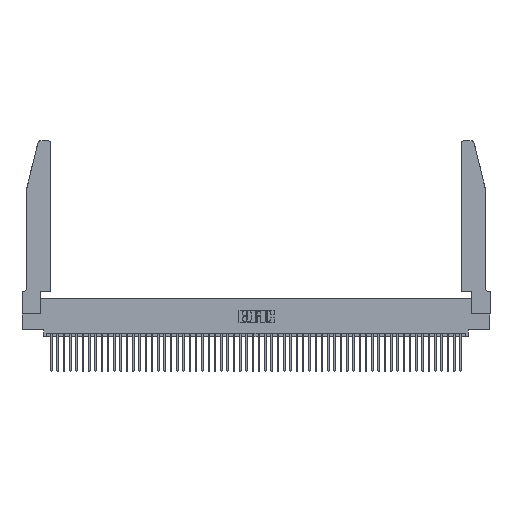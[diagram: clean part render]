
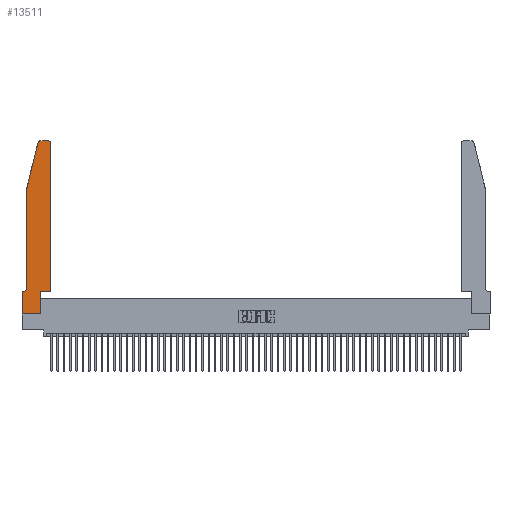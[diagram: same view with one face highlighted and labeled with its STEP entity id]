
A CAD part, top view. The second image highlights one B-rep face of the part: STEP entity #13511.
In plain terms, the highlighted planar face has unit normal (0, 0, 1).
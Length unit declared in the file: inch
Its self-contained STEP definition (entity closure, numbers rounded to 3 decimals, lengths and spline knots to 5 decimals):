
#61 = VECTOR ( 'NONE', #6870, 39.37008 ) ;
#768 = LINE ( 'NONE', #10422, #43506 ) ;
#879 = ORIENTED_EDGE ( 'NONE', *, *, #13769, .T. ) ;
#1245 = ORIENTED_EDGE ( 'NONE', *, *, #14559, .T. ) ;
#1617 = DIRECTION ( 'NONE',  ( 1., 0., 0. ) ) ;
#2369 = ORIENTED_EDGE ( 'NONE', *, *, #18976, .T. ) ;
#3714 = DIRECTION ( 'NONE',  ( 0., 0., 1. ) ) ;
#3869 = AXIS2_PLACEMENT_3D ( 'NONE', #19925, #40355, #28177 ) ;
#5569 = VERTEX_POINT ( 'NONE', #9003 ) ;
#6721 = VECTOR ( 'NONE', #52721, 39.37008 ) ;
#6870 = DIRECTION ( 'NONE',  ( -1., 0., 0. ) ) ;
#6979 = DIRECTION ( 'NONE',  ( -1., 0., 0. ) ) ;
#7592 = ORIENTED_EDGE ( 'NONE', *, *, #8691, .T. ) ;
#8308 = LINE ( 'NONE', #8914, #30263 ) ;
#8430 = VERTEX_POINT ( 'NONE', #43903 ) ;
#8691 = EDGE_CURVE ( 'NONE', #28145, #45264, #40369, .T. ) ;
#8846 = LINE ( 'NONE', #39069, #29527 ) ;
#8914 = CARTESIAN_POINT ( 'NONE',  ( 0.0755, 2., 0.37 ) ) ;
#9003 = CARTESIAN_POINT ( 'NONE',  ( 0.2865, 0.35, 0.37 ) ) ;
#9047 = CARTESIAN_POINT ( 'NONE',  ( 0.4505, 2.72, 0.37 ) ) ;
#9495 = CARTESIAN_POINT ( 'NONE',  ( 0., 0.35, 0.37 ) ) ;
#9639 = EDGE_CURVE ( 'NONE', #45264, #5569, #29175, .T. ) ;
#9743 = LINE ( 'NONE', #35895, #50912 ) ;
#10422 = CARTESIAN_POINT ( 'NONE',  ( 0.4505, 0.35, 0.37 ) ) ;
#11673 = ORIENTED_EDGE ( 'NONE', *, *, #46600, .T. ) ;
#11940 = VERTEX_POINT ( 'NONE', #47380 ) ;
#12599 = CARTESIAN_POINT ( 'NONE',  ( 0., 0., 0.37 ) ) ;
#13511 = ADVANCED_FACE ( 'NONE', ( #27551 ), #24076, .T. ) ;
#13596 = CARTESIAN_POINT ( 'NONE',  ( 0.4205, 2.75, 0.37 ) ) ;
#13769 = EDGE_CURVE ( 'NONE', #35258, #48527, #25578, .T. ) ;
#13972 = ORIENTED_EDGE ( 'NONE', *, *, #29061, .T. ) ;
#14559 = EDGE_CURVE ( 'NONE', #11940, #29943, #33227, .T. ) ;
#16245 = ORIENTED_EDGE ( 'NONE', *, *, #33513, .T. ) ;
#16617 = VERTEX_POINT ( 'NONE', #28194 ) ;
#18976 = EDGE_CURVE ( 'NONE', #5569, #47045, #8846, .T. ) ;
#18980 = EDGE_LOOP ( 'NONE', ( #22024, #879, #25818, #13972, #11673, #1245, #16245, #7592, #36953, #2369, #25454, #41870 ) ) ;
#19276 = CARTESIAN_POINT ( 'NONE',  ( 0.0755, 0.35, 0.37 ) ) ;
#19925 = CARTESIAN_POINT ( 'NONE',  ( 0., 0.35, 0.37 ) ) ;
#22024 = ORIENTED_EDGE ( 'NONE', *, *, #47142, .T. ) ;
#22861 = DIRECTION ( 'NONE',  ( 0., -1., 0. ) ) ;
#23502 = CARTESIAN_POINT ( 'NONE',  ( 0.284, 2.75, 0.37 ) ) ;
#23927 = CARTESIAN_POINT ( 'NONE',  ( 0.0755, 2., 0.37 ) ) ;
#24076 = PLANE ( 'NONE',  #3869 ) ;
#24662 = DIRECTION ( 'NONE',  ( 0., 0., -1. ) ) ;
#24849 = VERTEX_POINT ( 'NONE', #9047 ) ;
#25454 = ORIENTED_EDGE ( 'NONE', *, *, #25976, .T. ) ;
#25578 = CIRCLE ( 'NONE', #48164, 0.03 ) ;
#25818 = ORIENTED_EDGE ( 'NONE', *, *, #33214, .T. ) ;
#25976 = EDGE_CURVE ( 'NONE', #47045, #24849, #768, .T. ) ;
#26416 = DIRECTION ( 'NONE',  ( 0., 1., 0. ) ) ;
#26548 = DIRECTION ( 'NONE',  ( 0., 0., 1. ) ) ;
#26938 = CARTESIAN_POINT ( 'NONE',  ( 0.4505, 0.35, 0.37 ) ) ;
#27551 = FACE_OUTER_BOUND ( 'NONE', #18980, .T. ) ;
#28145 = VERTEX_POINT ( 'NONE', #46733 ) ;
#28177 = DIRECTION ( 'NONE',  ( 1., 0., 0. ) ) ;
#28194 = CARTESIAN_POINT ( 'NONE',  ( 0.0755, 2., 0.37 ) ) ;
#28344 = LINE ( 'NONE', #39157, #48823 ) ;
#28383 = CIRCLE ( 'NONE', #37856, 0.03 ) ;
#28613 = CARTESIAN_POINT ( 'NONE',  ( 0.4205, 2.72, 0.37 ) ) ;
#29061 = EDGE_CURVE ( 'NONE', #16617, #8430, #39667, .T. ) ;
#29175 = LINE ( 'NONE', #30515, #49674 ) ;
#29527 = VECTOR ( 'NONE', #43197, 39.37008 ) ;
#29943 = VERTEX_POINT ( 'NONE', #9495 ) ;
#30263 = VECTOR ( 'NONE', #37738, 39.37008 ) ;
#30515 = CARTESIAN_POINT ( 'NONE',  ( 0.2865, 0.35, 0.37 ) ) ;
#30732 = VECTOR ( 'NONE', #41384, 39.37008 ) ;
#32722 = DIRECTION ( 'NONE',  ( 1., 0., 0. ) ) ;
#33214 = EDGE_CURVE ( 'NONE', #48527, #16617, #8308, .T. ) ;
#33227 = LINE ( 'NONE', #19276, #61 ) ;
#33513 = EDGE_CURVE ( 'NONE', #29943, #28145, #28344, .T. ) ;
#34730 = AXIS2_PLACEMENT_3D ( 'NONE', #49165, #24662, #53288 ) ;
#35258 = VERTEX_POINT ( 'NONE', #23502 ) ;
#35895 = CARTESIAN_POINT ( 'NONE',  ( 0.2605, 2.75, 0.37 ) ) ;
#36121 = EDGE_CURVE ( 'NONE', #24849, #48796, #28383, .T. ) ;
#36953 = ORIENTED_EDGE ( 'NONE', *, *, #9639, .T. ) ;
#37738 = DIRECTION ( 'NONE',  ( -0.239, -0.971, 0. ) ) ;
#37856 = AXIS2_PLACEMENT_3D ( 'NONE', #28613, #3714, #32722 ) ;
#39069 = CARTESIAN_POINT ( 'NONE',  ( 0.4505, 0.35, 0.37 ) ) ;
#39157 = CARTESIAN_POINT ( 'NONE',  ( 0., 0., 0.37 ) ) ;
#39667 = LINE ( 'NONE', #23927, #6721 ) ;
#40355 = DIRECTION ( 'NONE',  ( 0., 0., 1. ) ) ;
#40369 = LINE ( 'NONE', #12599, #30732 ) ;
#41384 = DIRECTION ( 'NONE',  ( 1., 0., 0. ) ) ;
#41870 = ORIENTED_EDGE ( 'NONE', *, *, #36121, .T. ) ;
#43197 = DIRECTION ( 'NONE',  ( 1., 0., 0. ) ) ;
#43333 = DIRECTION ( 'NONE',  ( 0., 1., 0. ) ) ;
#43506 = VECTOR ( 'NONE', #43333, 39.37008 ) ;
#43903 = CARTESIAN_POINT ( 'NONE',  ( 0.0755, 0.42, 0.37 ) ) ;
#45264 = VERTEX_POINT ( 'NONE', #51182 ) ;
#46600 = EDGE_CURVE ( 'NONE', #8430, #11940, #53139, .T. ) ;
#46733 = CARTESIAN_POINT ( 'NONE',  ( 0., 0., 0.37 ) ) ;
#47045 = VERTEX_POINT ( 'NONE', #26938 ) ;
#47142 = EDGE_CURVE ( 'NONE', #48796, #35258, #9743, .T. ) ;
#47380 = CARTESIAN_POINT ( 'NONE',  ( 0.0055, 0.35, 0.37 ) ) ;
#48164 = AXIS2_PLACEMENT_3D ( 'NONE', #51060, #26548, #1617 ) ;
#48527 = VERTEX_POINT ( 'NONE', #53118 ) ;
#48796 = VERTEX_POINT ( 'NONE', #13596 ) ;
#48823 = VECTOR ( 'NONE', #22861, 39.37008 ) ;
#49165 = CARTESIAN_POINT ( 'NONE',  ( 0.0055, 0.42, 0.37 ) ) ;
#49674 = VECTOR ( 'NONE', #26416, 39.37008 ) ;
#50912 = VECTOR ( 'NONE', #6979, 39.37008 ) ;
#51060 = CARTESIAN_POINT ( 'NONE',  ( 0.284, 2.72, 0.37 ) ) ;
#51182 = CARTESIAN_POINT ( 'NONE',  ( 0.2865, 0., 0.37 ) ) ;
#52721 = DIRECTION ( 'NONE',  ( 0., -1., 0. ) ) ;
#53118 = CARTESIAN_POINT ( 'NONE',  ( 0.25487, 2.72718, 0.37 ) ) ;
#53139 = CIRCLE ( 'NONE', #34730, 0.07 ) ;
#53288 = DIRECTION ( 'NONE',  ( -1., 0., 0. ) ) ;
